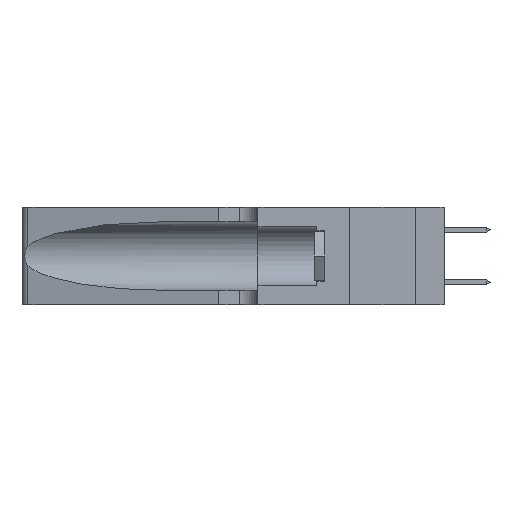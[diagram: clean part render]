
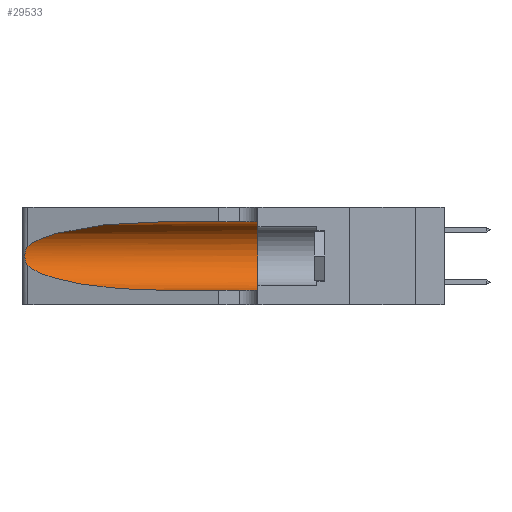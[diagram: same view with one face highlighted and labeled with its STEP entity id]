
A CAD part, left-side view. The second image highlights one B-rep face of the part: STEP entity #29533.
In plain terms, the highlighted cylindrical face has radius 3.308 mm (diameter 6.617 mm), a partial arc.
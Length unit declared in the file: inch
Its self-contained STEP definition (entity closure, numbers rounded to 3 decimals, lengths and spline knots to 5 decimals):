
#1529 = CARTESIAN_POINT ( 'NONE',  ( 0.26018, 1.23835, 0.19895 ) ) ;
#2074 = CARTESIAN_POINT ( 'NONE',  ( 0.1305, 0.72297, 0.05475 ) ) ;
#3415 = AXIS2_PLACEMENT_3D ( 'NONE', #11532, #4324, #16235 ) ;
#3919 = DIRECTION ( 'NONE',  ( 0., -1., 0. ) ) ;
#3929 = CARTESIAN_POINT ( 'NONE',  ( 0.26075, 1.23896, 0.178 ) ) ;
#4324 = DIRECTION ( 'NONE',  ( 0., -1., 0. ) ) ;
#4503 = CARTESIAN_POINT ( 'NONE',  ( 0.18966, 0.96281, 0.05475 ) ) ;
#5263 = CARTESIAN_POINT ( 'NONE',  ( 0.1305, 0.35, 0.185 ) ) ;
#5486 = EDGE_CURVE ( 'NONE', #9732, #29016, #25138, .T. ) ;
#6131 = ORIENTED_EDGE ( 'NONE', *, *, #22639, .T. ) ;
#6302 = CARTESIAN_POINT ( 'NONE',  ( 0.25856, 1.23593, 0.16098 ) ) ;
#6558 = CARTESIAN_POINT ( 'NONE',  ( 0.1305, 0.72297, 0.31525 ) ) ;
#6887 = CARTESIAN_POINT ( 'NONE',  ( 0.25487, 1.22718, 0.14631 ) ) ;
#7204 = CARTESIAN_POINT ( 'NONE',  ( 0.25487, 1.22718, 0.22369 ) ) ;
#7662 = DIRECTION ( 'NONE',  ( 0., 0., 1. ) ) ;
#8728 = CARTESIAN_POINT ( 'NONE',  ( 0.25639, 1.23186, 0.15144 ) ) ;
#8998 = CARTESIAN_POINT ( 'NONE',  ( 0.18966, 0.96281, 0.31525 ) ) ;
#9162 = CARTESIAN_POINT ( 'NONE',  ( 0.1305, 0.35, 0.31525 ) ) ;
#9321 = CARTESIAN_POINT ( 'NONE',  ( 0.1305, 0.72297, 0.05475 ) ) ;
#9632 = CARTESIAN_POINT ( 'NONE',  ( 0.25555, 1.22994, 0.2215 ) ) ;
#9732 = VERTEX_POINT ( 'NONE', #18772 ) ;
#9840 = CYLINDRICAL_SURFACE ( 'NONE', #3415, 0.13025 ) ;
#10577 = FACE_OUTER_BOUND ( 'NONE', #16577, .T. ) ;
#11061 = EDGE_CURVE ( 'NONE', #17840, #13390, #29742, .T. ) ;
#11114 = CARTESIAN_POINT ( 'NONE',  ( 0.25487, 1.22718, 0.14631 ) ) ;
#11382 = CARTESIAN_POINT ( 'NONE',  ( 0.25487, 1.22718, 0.22369 ) ) ;
#11390 = EDGE_CURVE ( 'NONE', #29803, #17840, #19087, .T. ) ;
#11532 = CARTESIAN_POINT ( 'NONE',  ( 0.1305, 1.61858, 0.185 ) ) ;
#12878 = EDGE_CURVE ( 'NONE', #29016, #13390, #24000, .T. ) ;
#13005 = DIRECTION ( 'NONE',  ( 0., -1., 0. ) ) ;
#13390 = VERTEX_POINT ( 'NONE', #14234 ) ;
#13448 = CARTESIAN_POINT ( 'NONE',  ( 0.25639, 1.23184, 0.21858 ) ) ;
#13935 = ORIENTED_EDGE ( 'NONE', *, *, #11061, .T. ) ;
#14234 = CARTESIAN_POINT ( 'NONE',  ( 0.1305, 0.35, 0.05475 ) ) ;
#14400 = VERTEX_POINT ( 'NONE', #16641 ) ;
#14744 =( BOUNDED_CURVE ( )  B_SPLINE_CURVE ( 3, ( #6558, #8998, #25587, #11382 ),
 .UNSPECIFIED., .F., .F. ) 
 B_SPLINE_CURVE_WITH_KNOTS ( ( 4, 4 ),
 ( 1.5708, 2.84003 ),
 .UNSPECIFIED. ) 
 CURVE ( )  GEOMETRIC_REPRESENTATION_ITEM ( )  RATIONAL_B_SPLINE_CURVE ( ( 1., 0.87, 0.87, 1. ) ) 
 REPRESENTATION_ITEM ( '' )  );
#15834 = CARTESIAN_POINT ( 'NONE',  ( 0.25854, 1.2359, 0.20912 ) ) ;
#16235 = DIRECTION ( 'NONE',  ( 0., 0., -1. ) ) ;
#16293 = B_SPLINE_CURVE_WITH_KNOTS ( 'NONE', 3,
 ( #7204, #9632, #13448, #30050, #15834, #1529, #18207, #3929, #20573, #6302, #22943, #8728, #25317, #11114 ),
 .UNSPECIFIED., .F., .F.,
 ( 4, 2, 2, 2, 2, 2, 4 ),
 ( 0., 0.00027, 0.00053, 0.00107, 0.0016, 0.00187, 0.00214 ),
 .UNSPECIFIED. ) ;
#16577 = EDGE_LOOP ( 'NONE', ( #26690, #6131, #22184, #13935, #23596, #28230 ) ) ;
#16641 = CARTESIAN_POINT ( 'NONE',  ( 0.25487, 1.22718, 0.22369 ) ) ;
#17772 = CARTESIAN_POINT ( 'NONE',  ( 0.1305, 1.61858, 0.05475 ) ) ;
#17840 = VERTEX_POINT ( 'NONE', #2074 ) ;
#18207 = CARTESIAN_POINT ( 'NONE',  ( 0.26075, 1.23896, 0.19203 ) ) ;
#18772 = CARTESIAN_POINT ( 'NONE',  ( 0.1305, 0.72297, 0.31525 ) ) ;
#19087 =( BOUNDED_CURVE ( )  B_SPLINE_CURVE ( 3, ( #6887, #21156, #4503, #9321 ),
 .UNSPECIFIED., .F., .F. ) 
 B_SPLINE_CURVE_WITH_KNOTS ( ( 4, 4 ),
 ( 3.44316, 4.71239 ),
 .UNSPECIFIED. ) 
 CURVE ( )  GEOMETRIC_REPRESENTATION_ITEM ( )  RATIONAL_B_SPLINE_CURVE ( ( 1., 0.87, 0.87, 1. ) ) 
 REPRESENTATION_ITEM ( '' )  );
#20258 = AXIS2_PLACEMENT_3D ( 'NONE', #5263, #21895, #7662 ) ;
#20573 = CARTESIAN_POINT ( 'NONE',  ( 0.26017, 1.23833, 0.17102 ) ) ;
#21156 = CARTESIAN_POINT ( 'NONE',  ( 0.2373, 1.15595, 0.08982 ) ) ;
#21895 = DIRECTION ( 'NONE',  ( 0., 1., 0. ) ) ;
#22184 = ORIENTED_EDGE ( 'NONE', *, *, #11390, .T. ) ;
#22639 = EDGE_CURVE ( 'NONE', #14400, #29803, #16293, .T. ) ;
#22935 = CARTESIAN_POINT ( 'NONE',  ( 0.1305, 1.61858, 0.31525 ) ) ;
#22943 = CARTESIAN_POINT ( 'NONE',  ( 0.25789, 1.23486, 0.15765 ) ) ;
#23384 = VECTOR ( 'NONE', #13005, 39.37008 ) ;
#23596 = ORIENTED_EDGE ( 'NONE', *, *, #12878, .F. ) ;
#24000 = CIRCLE ( 'NONE', #20258, 0.13025 ) ;
#24394 = VECTOR ( 'NONE', #3919, 39.37008 ) ;
#25138 = LINE ( 'NONE', #22935, #24394 ) ;
#25317 = CARTESIAN_POINT ( 'NONE',  ( 0.25555, 1.22993, 0.14849 ) ) ;
#25587 = CARTESIAN_POINT ( 'NONE',  ( 0.2373, 1.15595, 0.28018 ) ) ;
#26690 = ORIENTED_EDGE ( 'NONE', *, *, #30153, .T. ) ;
#28230 = ORIENTED_EDGE ( 'NONE', *, *, #5486, .F. ) ;
#29016 = VERTEX_POINT ( 'NONE', #9162 ) ;
#29181 = CARTESIAN_POINT ( 'NONE',  ( 0.25487, 1.22718, 0.14631 ) ) ;
#29533 = ADVANCED_FACE ( 'NONE', ( #10577 ), #9840, .F. ) ;
#29742 = LINE ( 'NONE', #17772, #23384 ) ;
#29803 = VERTEX_POINT ( 'NONE', #29181 ) ;
#30050 = CARTESIAN_POINT ( 'NONE',  ( 0.25787, 1.23484, 0.2124 ) ) ;
#30153 = EDGE_CURVE ( 'NONE', #9732, #14400, #14744, .T. ) ;
